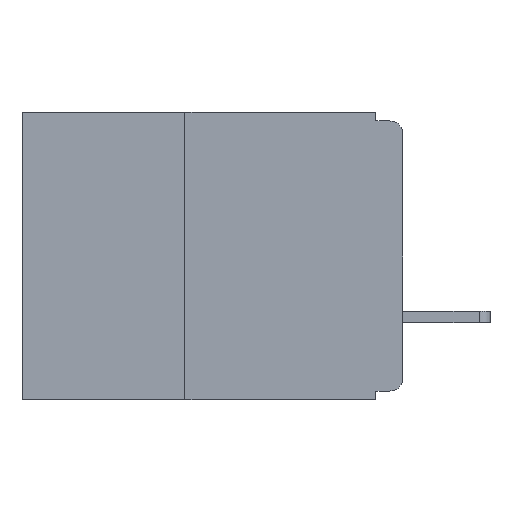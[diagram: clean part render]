
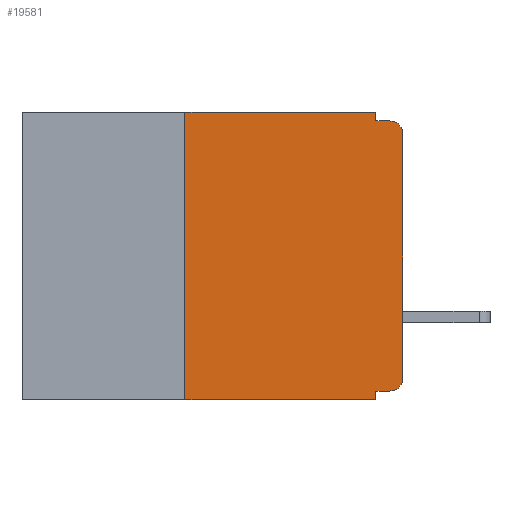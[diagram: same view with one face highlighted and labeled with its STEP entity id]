
A CAD part, left-side view. The second image highlights one B-rep face of the part: STEP entity #19581.
In plain terms, the highlighted planar face has unit normal (-1, 0, 0).
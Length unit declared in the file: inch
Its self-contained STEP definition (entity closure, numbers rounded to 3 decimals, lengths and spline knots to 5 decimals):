
#167 = DIRECTION ( 'NONE',  ( 0., -1., 0. ) ) ;
#320 = ORIENTED_EDGE ( 'NONE', *, *, #17405, .T. ) ;
#776 = DIRECTION ( 'NONE',  ( 0., 1., 0. ) ) ;
#784 = DIRECTION ( 'NONE',  ( 0., 0., 1. ) ) ;
#989 = FACE_OUTER_BOUND ( 'NONE', #8163, .T. ) ;
#1477 = DIRECTION ( 'NONE',  ( 1., 0., 0. ) ) ;
#1687 = CARTESIAN_POINT ( 'NONE',  ( 0., 0.031, -0.32 ) ) ;
#1732 = CARTESIAN_POINT ( 'NONE',  ( 0., 0.031, 0. ) ) ;
#1922 = VECTOR ( 'NONE', #10192, 39.37008 ) ;
#2123 = LINE ( 'NONE', #7925, #13725 ) ;
#2222 = EDGE_CURVE ( 'NONE', #19189, #4294, #5852, .T. ) ;
#2374 = CARTESIAN_POINT ( 'NONE',  ( 0., 0., -0.01 ) ) ;
#2573 = ORIENTED_EDGE ( 'NONE', *, *, #14507, .T. ) ;
#2617 = VECTOR ( 'NONE', #17232, 39.37008 ) ;
#2674 = CARTESIAN_POINT ( 'NONE',  ( 0., 0.031, -0.33 ) ) ;
#3966 = EDGE_CURVE ( 'NONE', #5348, #13235, #18829, .T. ) ;
#4251 = DIRECTION ( 'NONE',  ( 0., 0., -1. ) ) ;
#4294 = VERTEX_POINT ( 'NONE', #13392 ) ;
#4797 = DIRECTION ( 'NONE',  ( 0., 0., -1. ) ) ;
#5001 = EDGE_CURVE ( 'NONE', #12495, #8205, #5056, .T. ) ;
#5056 = LINE ( 'NONE', #5177, #16505 ) ;
#5133 = EDGE_CURVE ( 'NONE', #13235, #12495, #6211, .T. ) ;
#5177 = CARTESIAN_POINT ( 'NONE',  ( 0., 0.031, 0. ) ) ;
#5348 = VERTEX_POINT ( 'NONE', #10193 ) ;
#5436 = CARTESIAN_POINT ( 'NONE',  ( 0., 0., 0. ) ) ;
#5792 = VECTOR ( 'NONE', #11450, 39.37008 ) ;
#5852 = CIRCLE ( 'NONE', #15331, 0.015 ) ;
#5870 = VECTOR ( 'NONE', #784, 39.37008 ) ;
#6091 = PLANE ( 'NONE',  #13584 ) ;
#6211 = LINE ( 'NONE', #17305, #2617 ) ;
#6708 = CARTESIAN_POINT ( 'NONE',  ( 0., 0.015, -0.305 ) ) ;
#6811 = VERTEX_POINT ( 'NONE', #11873 ) ;
#6991 = VECTOR ( 'NONE', #12465, 39.37008 ) ;
#7036 = CARTESIAN_POINT ( 'NONE',  ( 0., 0.015, -0.025 ) ) ;
#7911 = EDGE_CURVE ( 'NONE', #8205, #4294, #10288, .T. ) ;
#7925 = CARTESIAN_POINT ( 'NONE',  ( 0., 0.437, -0.33 ) ) ;
#8018 = VERTEX_POINT ( 'NONE', #13213 ) ;
#8163 = EDGE_LOOP ( 'NONE', ( #2573, #10637, #15038, #18975, #11573, #15984, #320, #9047, #12971, #16936 ) ) ;
#8205 = VERTEX_POINT ( 'NONE', #13737 ) ;
#8233 = DIRECTION ( 'NONE',  ( 0., 0., -1. ) ) ;
#8739 = CARTESIAN_POINT ( 'NONE',  ( 0., 0.25, -0.33 ) ) ;
#9047 = ORIENTED_EDGE ( 'NONE', *, *, #16370, .F. ) ;
#9325 = CIRCLE ( 'NONE', #14791, 0.015 ) ;
#9434 = CARTESIAN_POINT ( 'NONE',  ( 0., 0., -0.025 ) ) ;
#9603 = LINE ( 'NONE', #2674, #1922 ) ;
#9915 = LINE ( 'NONE', #5436, #5870 ) ;
#10192 = DIRECTION ( 'NONE',  ( 0., 0., -1. ) ) ;
#10193 = CARTESIAN_POINT ( 'NONE',  ( 0., 0.25, -0.33 ) ) ;
#10288 = LINE ( 'NONE', #2374, #5792 ) ;
#10637 = ORIENTED_EDGE ( 'NONE', *, *, #2222, .T. ) ;
#11143 = CARTESIAN_POINT ( 'NONE',  ( 0., 0.25, 0. ) ) ;
#11450 = DIRECTION ( 'NONE',  ( 0., -1., 0. ) ) ;
#11566 = LINE ( 'NONE', #15871, #15031 ) ;
#11573 = ORIENTED_EDGE ( 'NONE', *, *, #5133, .F. ) ;
#11873 = CARTESIAN_POINT ( 'NONE',  ( 0., 0., -0.305 ) ) ;
#12114 = DIRECTION ( 'NONE',  ( 0., 0., -1. ) ) ;
#12465 = DIRECTION ( 'NONE',  ( 0., 0., 1. ) ) ;
#12495 = VERTEX_POINT ( 'NONE', #1732 ) ;
#12773 = DIRECTION ( 'NONE',  ( -1., 0., 0. ) ) ;
#12971 = ORIENTED_EDGE ( 'NONE', *, *, #13374, .F. ) ;
#13213 = CARTESIAN_POINT ( 'NONE',  ( 0., 0.015, -0.32 ) ) ;
#13235 = VERTEX_POINT ( 'NONE', #11143 ) ;
#13374 = EDGE_CURVE ( 'NONE', #8018, #16590, #11566, .T. ) ;
#13392 = CARTESIAN_POINT ( 'NONE',  ( 0., 0.015, -0.01 ) ) ;
#13584 = AXIS2_PLACEMENT_3D ( 'NONE', #18068, #1477, #12114 ) ;
#13725 = VECTOR ( 'NONE', #167, 39.37008 ) ;
#13737 = CARTESIAN_POINT ( 'NONE',  ( 0., 0.031, -0.01 ) ) ;
#14390 = VERTEX_POINT ( 'NONE', #15686 ) ;
#14507 = EDGE_CURVE ( 'NONE', #6811, #19189, #9915, .T. ) ;
#14791 = AXIS2_PLACEMENT_3D ( 'NONE', #6708, #17140, #8233 ) ;
#15031 = VECTOR ( 'NONE', #776, 39.37008 ) ;
#15038 = ORIENTED_EDGE ( 'NONE', *, *, #7911, .F. ) ;
#15331 = AXIS2_PLACEMENT_3D ( 'NONE', #7036, #12773, #4797 ) ;
#15686 = CARTESIAN_POINT ( 'NONE',  ( 0., 0.031, -0.33 ) ) ;
#15871 = CARTESIAN_POINT ( 'NONE',  ( 0., 0., -0.32 ) ) ;
#15984 = ORIENTED_EDGE ( 'NONE', *, *, #3966, .F. ) ;
#16370 = EDGE_CURVE ( 'NONE', #16590, #14390, #9603, .T. ) ;
#16505 = VECTOR ( 'NONE', #4251, 39.37008 ) ;
#16590 = VERTEX_POINT ( 'NONE', #1687 ) ;
#16936 = ORIENTED_EDGE ( 'NONE', *, *, #18119, .T. ) ;
#17140 = DIRECTION ( 'NONE',  ( -1., 0., 0. ) ) ;
#17232 = DIRECTION ( 'NONE',  ( 0., -1., 0. ) ) ;
#17305 = CARTESIAN_POINT ( 'NONE',  ( 0., 0.437, 0. ) ) ;
#17405 = EDGE_CURVE ( 'NONE', #5348, #14390, #2123, .T. ) ;
#18068 = CARTESIAN_POINT ( 'NONE',  ( 0., 0.437, 0. ) ) ;
#18119 = EDGE_CURVE ( 'NONE', #8018, #6811, #9325, .T. ) ;
#18829 = LINE ( 'NONE', #8739, #6991 ) ;
#18975 = ORIENTED_EDGE ( 'NONE', *, *, #5001, .F. ) ;
#19189 = VERTEX_POINT ( 'NONE', #9434 ) ;
#19581 = ADVANCED_FACE ( 'NONE', ( #989 ), #6091, .F. ) ;
